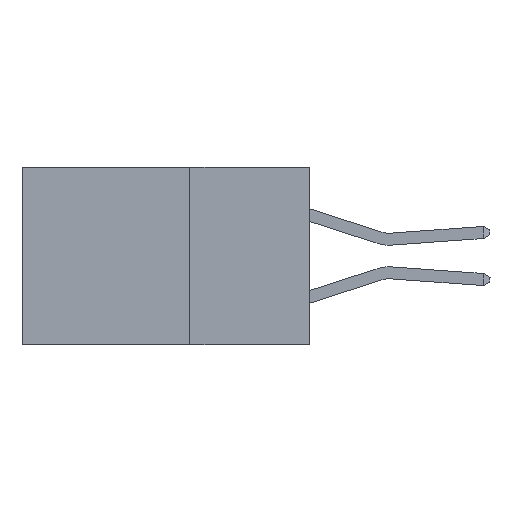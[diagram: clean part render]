
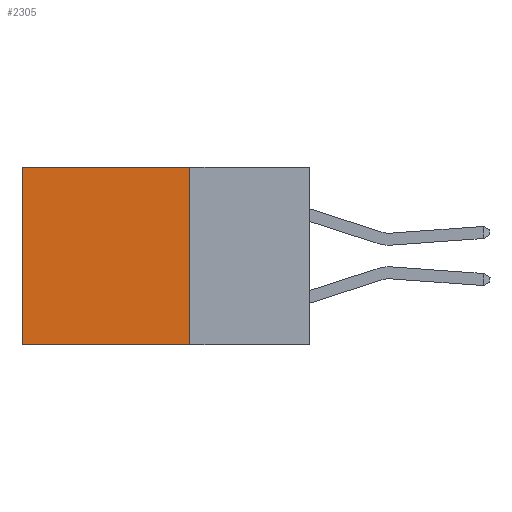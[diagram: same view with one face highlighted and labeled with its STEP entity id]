
A CAD part, left-side view. The second image highlights one B-rep face of the part: STEP entity #2305.
In plain terms, the highlighted planar face has unit normal (-1, 0, 0).
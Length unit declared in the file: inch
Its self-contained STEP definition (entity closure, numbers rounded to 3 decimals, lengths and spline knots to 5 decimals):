
#44 = LINE ( 'NONE', #2092, #7599 ) ;
#77 = CARTESIAN_POINT ( 'NONE',  ( 0.2615, 0.6, -0.37 ) ) ;
#531 = DIRECTION ( 'NONE',  ( 0., 1., 0. ) ) ;
#645 = LINE ( 'NONE', #6909, #8601 ) ;
#1194 = VERTEX_POINT ( 'NONE', #7542 ) ;
#1342 = CARTESIAN_POINT ( 'NONE',  ( 0.2615, 0.25, -0.37 ) ) ;
#1428 = CARTESIAN_POINT ( 'NONE',  ( 0.2615, 0.25, -0.37 ) ) ;
#1798 = VECTOR ( 'NONE', #531, 39.37008 ) ;
#1889 = ORIENTED_EDGE ( 'NONE', *, *, #2331, .F. ) ;
#1904 = ORIENTED_EDGE ( 'NONE', *, *, #3978, .T. ) ;
#2079 = CARTESIAN_POINT ( 'NONE',  ( 0.2615, 0.25, -0.37 ) ) ;
#2092 = CARTESIAN_POINT ( 'NONE',  ( 0.2615, 0.25, 0. ) ) ;
#2254 = ORIENTED_EDGE ( 'NONE', *, *, #7475, .T. ) ;
#2305 = ADVANCED_FACE ( 'NONE', ( #4231 ), #7403, .F. ) ;
#2331 = EDGE_CURVE ( 'NONE', #10542, #10602, #8080, .T. ) ;
#2609 = EDGE_LOOP ( 'NONE', ( #1904, #7443, #1889, #2254 ) ) ;
#2630 = DIRECTION ( 'NONE',  ( 0., 0., -1. ) ) ;
#3133 = DIRECTION ( 'NONE',  ( 1., 0., 0. ) ) ;
#3978 = EDGE_CURVE ( 'NONE', #1194, #4781, #645, .T. ) ;
#4231 = FACE_OUTER_BOUND ( 'NONE', #2609, .T. ) ;
#4744 = DIRECTION ( 'NONE',  ( 0., 1., 0. ) ) ;
#4781 = VERTEX_POINT ( 'NONE', #77 ) ;
#4942 = CARTESIAN_POINT ( 'NONE',  ( 0.2615, 0.25, -0.37 ) ) ;
#6161 = AXIS2_PLACEMENT_3D ( 'NONE', #1342, #3133, #9241 ) ;
#6909 = CARTESIAN_POINT ( 'NONE',  ( 0.2615, 0.6, -0.37 ) ) ;
#7403 = PLANE ( 'NONE',  #6161 ) ;
#7443 = ORIENTED_EDGE ( 'NONE', *, *, #9482, .F. ) ;
#7475 = EDGE_CURVE ( 'NONE', #10542, #1194, #44, .T. ) ;
#7542 = CARTESIAN_POINT ( 'NONE',  ( 0.2615, 0.6, 0. ) ) ;
#7599 = VECTOR ( 'NONE', #4744, 39.37008 ) ;
#8080 = LINE ( 'NONE', #1428, #10275 ) ;
#8601 = VECTOR ( 'NONE', #2630, 39.37008 ) ;
#8782 = LINE ( 'NONE', #4942, #1798 ) ;
#9241 = DIRECTION ( 'NONE',  ( 0., 0., -1. ) ) ;
#9319 = DIRECTION ( 'NONE',  ( 0., 0., -1. ) ) ;
#9482 = EDGE_CURVE ( 'NONE', #10602, #4781, #8782, .T. ) ;
#9745 = CARTESIAN_POINT ( 'NONE',  ( 0.2615, 0.25, 0. ) ) ;
#10275 = VECTOR ( 'NONE', #9319, 39.37008 ) ;
#10542 = VERTEX_POINT ( 'NONE', #9745 ) ;
#10602 = VERTEX_POINT ( 'NONE', #2079 ) ;
